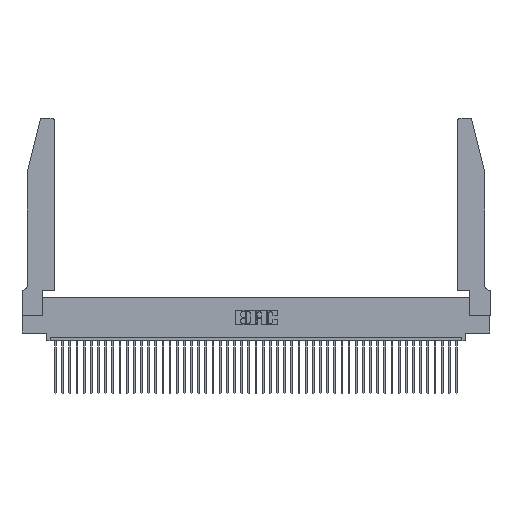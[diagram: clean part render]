
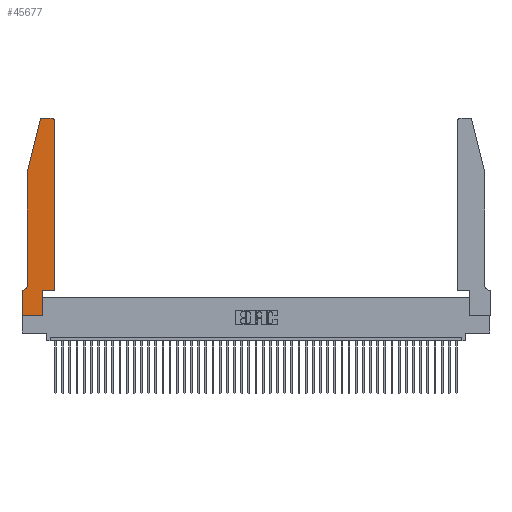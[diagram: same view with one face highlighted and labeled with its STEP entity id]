
A CAD part, top view. The second image highlights one B-rep face of the part: STEP entity #45677.
In plain terms, the highlighted planar face has unit normal (0, 0, 1).
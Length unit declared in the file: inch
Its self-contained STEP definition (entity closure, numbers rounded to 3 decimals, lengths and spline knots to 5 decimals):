
#329 = VECTOR ( 'NONE', #40037, 39.37008 ) ;
#835 = DIRECTION ( 'NONE',  ( 1., 0., 0. ) ) ;
#1162 = VECTOR ( 'NONE', #23060, 39.37008 ) ;
#1340 = CARTESIAN_POINT ( 'NONE',  ( 0.4505, 2.72, 0.37 ) ) ;
#2674 = CARTESIAN_POINT ( 'NONE',  ( 0.2865, 0.35, 0.37 ) ) ;
#3035 = CARTESIAN_POINT ( 'NONE',  ( 0.0055, 0.35, 0.37 ) ) ;
#3531 = VECTOR ( 'NONE', #38115, 39.37008 ) ;
#3575 = AXIS2_PLACEMENT_3D ( 'NONE', #19903, #26708, #40951 ) ;
#3887 = DIRECTION ( 'NONE',  ( 0., 0., -1. ) ) ;
#4569 = CARTESIAN_POINT ( 'NONE',  ( 0.4205, 2.75, 0.37 ) ) ;
#4655 = CARTESIAN_POINT ( 'NONE',  ( 0., 0., 0.37 ) ) ;
#5212 = LINE ( 'NONE', #35551, #31219 ) ;
#5347 = ORIENTED_EDGE ( 'NONE', *, *, #18317, .T. ) ;
#6349 = EDGE_CURVE ( 'NONE', #31987, #32236, #34155, .T. ) ;
#6745 = EDGE_CURVE ( 'NONE', #7110, #39506, #26875, .T. ) ;
#7110 = VERTEX_POINT ( 'NONE', #12346 ) ;
#7228 = CIRCLE ( 'NONE', #35115, 0.03 ) ;
#7332 = EDGE_CURVE ( 'NONE', #16633, #31987, #14613, .T. ) ;
#7805 = ORIENTED_EDGE ( 'NONE', *, *, #7332, .T. ) ;
#7959 = CARTESIAN_POINT ( 'NONE',  ( 0.2865, 0.35, 0.37 ) ) ;
#10338 = CARTESIAN_POINT ( 'NONE',  ( 0.2865, 0., 0.37 ) ) ;
#12008 = CARTESIAN_POINT ( 'NONE',  ( 0., 0.35, 0.37 ) ) ;
#12346 = CARTESIAN_POINT ( 'NONE',  ( 0.4505, 0.35, 0.37 ) ) ;
#13363 = CIRCLE ( 'NONE', #38043, 0.03 ) ;
#13691 = DIRECTION ( 'NONE',  ( 0., 0., 1. ) ) ;
#14613 = LINE ( 'NONE', #30553, #27892 ) ;
#14654 = ORIENTED_EDGE ( 'NONE', *, *, #43372, .T. ) ;
#14674 = EDGE_LOOP ( 'NONE', ( #5347, #25274, #35200, #44382, #44157, #7805, #14823, #31405, #14654, #21954, #33074, #29701 ) ) ;
#14823 = ORIENTED_EDGE ( 'NONE', *, *, #6349, .T. ) ;
#14835 = CARTESIAN_POINT ( 'NONE',  ( 0.4205, 2.72, 0.37 ) ) ;
#15223 = CARTESIAN_POINT ( 'NONE',  ( 0.284, 2.75, 0.37 ) ) ;
#15588 = CARTESIAN_POINT ( 'NONE',  ( 0.0755, 0.42, 0.37 ) ) ;
#15857 = VERTEX_POINT ( 'NONE', #7959 ) ;
#15909 = CARTESIAN_POINT ( 'NONE',  ( 0.2605, 2.75, 0.37 ) ) ;
#16633 = VERTEX_POINT ( 'NONE', #3035 ) ;
#17265 = VERTEX_POINT ( 'NONE', #15223 ) ;
#17702 = VERTEX_POINT ( 'NONE', #4569 ) ;
#17999 = DIRECTION ( 'NONE',  ( 0., 1., 0. ) ) ;
#18317 = EDGE_CURVE ( 'NONE', #17702, #17265, #28758, .T. ) ;
#18658 = DIRECTION ( 'NONE',  ( -1., 0., 0. ) ) ;
#19433 = CARTESIAN_POINT ( 'NONE',  ( 0.4505, 0.35, 0.37 ) ) ;
#19457 = CARTESIAN_POINT ( 'NONE',  ( 0.0755, 2., 0.37 ) ) ;
#19665 = DIRECTION ( 'NONE',  ( -1., 0., 0. ) ) ;
#19903 = CARTESIAN_POINT ( 'NONE',  ( 0., 0.35, 0.37 ) ) ;
#20222 = PLANE ( 'NONE',  #3575 ) ;
#21788 = CARTESIAN_POINT ( 'NONE',  ( 0.25487, 2.72718, 0.37 ) ) ;
#21954 = ORIENTED_EDGE ( 'NONE', *, *, #23573, .T. ) ;
#22256 = LINE ( 'NONE', #30849, #3531 ) ;
#22346 = VECTOR ( 'NONE', #42081, 39.37008 ) ;
#22389 = EDGE_CURVE ( 'NONE', #32236, #32743, #5212, .T. ) ;
#23060 = DIRECTION ( 'NONE',  ( -1., 0., 0. ) ) ;
#23117 = EDGE_CURVE ( 'NONE', #17265, #29815, #7228, .T. ) ;
#23573 = EDGE_CURVE ( 'NONE', #15857, #7110, #35428, .T. ) ;
#23727 = EDGE_CURVE ( 'NONE', #23829, #16633, #33168, .T. ) ;
#23829 = VERTEX_POINT ( 'NONE', #15588 ) ;
#24304 = VECTOR ( 'NONE', #35604, 39.37008 ) ;
#24755 = CARTESIAN_POINT ( 'NONE',  ( 0.0755, 2., 0.37 ) ) ;
#25274 = ORIENTED_EDGE ( 'NONE', *, *, #23117, .T. ) ;
#25480 = DIRECTION ( 'NONE',  ( 0., 0., 1. ) ) ;
#25924 = VECTOR ( 'NONE', #35755, 39.37008 ) ;
#26708 = DIRECTION ( 'NONE',  ( 0., 0., 1. ) ) ;
#26875 = LINE ( 'NONE', #19433, #29615 ) ;
#27892 = VECTOR ( 'NONE', #19665, 39.37008 ) ;
#28758 = LINE ( 'NONE', #15909, #1162 ) ;
#29615 = VECTOR ( 'NONE', #17999, 39.37008 ) ;
#29701 = ORIENTED_EDGE ( 'NONE', *, *, #39324, .T. ) ;
#29815 = VERTEX_POINT ( 'NONE', #21788 ) ;
#30553 = CARTESIAN_POINT ( 'NONE',  ( 0.0755, 0.35, 0.37 ) ) ;
#30849 = CARTESIAN_POINT ( 'NONE',  ( 0.0755, 2., 0.37 ) ) ;
#31219 = VECTOR ( 'NONE', #835, 39.37008 ) ;
#31405 = ORIENTED_EDGE ( 'NONE', *, *, #22389, .T. ) ;
#31502 = LINE ( 'NONE', #24755, #24304 ) ;
#31987 = VERTEX_POINT ( 'NONE', #12008 ) ;
#32176 = CARTESIAN_POINT ( 'NONE',  ( 0.0055, 0.42, 0.37 ) ) ;
#32236 = VERTEX_POINT ( 'NONE', #33829 ) ;
#32743 = VERTEX_POINT ( 'NONE', #10338 ) ;
#32934 = CARTESIAN_POINT ( 'NONE',  ( 0.4505, 0.35, 0.37 ) ) ;
#33074 = ORIENTED_EDGE ( 'NONE', *, *, #6745, .T. ) ;
#33168 = CIRCLE ( 'NONE', #39414, 0.07 ) ;
#33829 = CARTESIAN_POINT ( 'NONE',  ( 0., 0., 0.37 ) ) ;
#34155 = LINE ( 'NONE', #4655, #329 ) ;
#34932 = FACE_OUTER_BOUND ( 'NONE', #14674, .T. ) ;
#35115 = AXIS2_PLACEMENT_3D ( 'NONE', #39925, #13691, #41825 ) ;
#35200 = ORIENTED_EDGE ( 'NONE', *, *, #40855, .T. ) ;
#35428 = LINE ( 'NONE', #32934, #25924 ) ;
#35551 = CARTESIAN_POINT ( 'NONE',  ( 0., 0., 0.37 ) ) ;
#35604 = DIRECTION ( 'NONE',  ( -0.239, -0.971, 0. ) ) ;
#35755 = DIRECTION ( 'NONE',  ( 1., 0., 0. ) ) ;
#35904 = DIRECTION ( 'NONE',  ( 1., 0., 0. ) ) ;
#38043 = AXIS2_PLACEMENT_3D ( 'NONE', #14835, #25480, #35904 ) ;
#38115 = DIRECTION ( 'NONE',  ( 0., -1., 0. ) ) ;
#39324 = EDGE_CURVE ( 'NONE', #39506, #17702, #13363, .T. ) ;
#39414 = AXIS2_PLACEMENT_3D ( 'NONE', #32176, #3887, #18658 ) ;
#39506 = VERTEX_POINT ( 'NONE', #1340 ) ;
#39925 = CARTESIAN_POINT ( 'NONE',  ( 0.284, 2.72, 0.37 ) ) ;
#40037 = DIRECTION ( 'NONE',  ( 0., -1., 0. ) ) ;
#40855 = EDGE_CURVE ( 'NONE', #29815, #42959, #31502, .T. ) ;
#40951 = DIRECTION ( 'NONE',  ( 1., 0., 0. ) ) ;
#41210 = LINE ( 'NONE', #2674, #22346 ) ;
#41825 = DIRECTION ( 'NONE',  ( 1., 0., 0. ) ) ;
#42081 = DIRECTION ( 'NONE',  ( 0., 1., 0. ) ) ;
#42959 = VERTEX_POINT ( 'NONE', #19457 ) ;
#43372 = EDGE_CURVE ( 'NONE', #32743, #15857, #41210, .T. ) ;
#44157 = ORIENTED_EDGE ( 'NONE', *, *, #23727, .T. ) ;
#44382 = ORIENTED_EDGE ( 'NONE', *, *, #44508, .T. ) ;
#44508 = EDGE_CURVE ( 'NONE', #42959, #23829, #22256, .T. ) ;
#45677 = ADVANCED_FACE ( 'NONE', ( #34932 ), #20222, .T. ) ;
